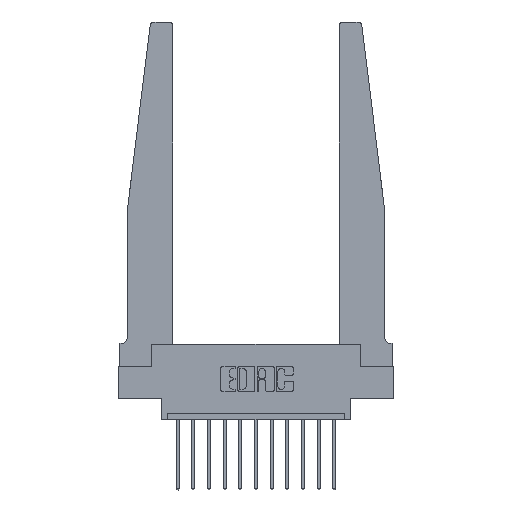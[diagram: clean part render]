
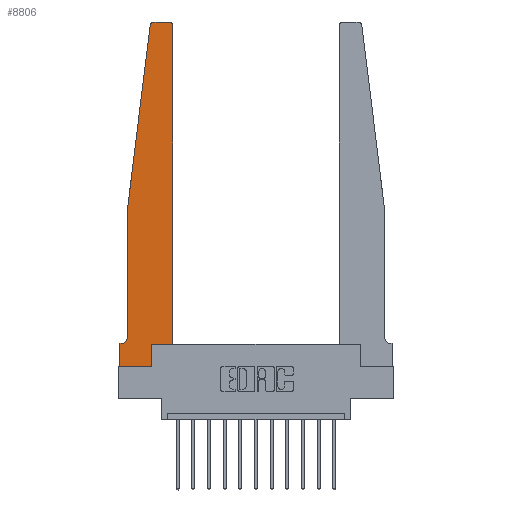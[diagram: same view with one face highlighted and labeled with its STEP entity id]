
A CAD part, top view. The second image highlights one B-rep face of the part: STEP entity #8806.
In plain terms, the highlighted planar face has unit normal (0, 0, 1).
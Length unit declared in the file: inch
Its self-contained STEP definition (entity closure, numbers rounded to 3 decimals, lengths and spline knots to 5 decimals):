
#67 = DIRECTION ( 'NONE',  ( 0., 0., -1. ) ) ;
#358 = CARTESIAN_POINT ( 'NONE',  ( 0.065, 1.25, 0.37 ) ) ;
#398 = CIRCLE ( 'NONE', #5786, 0.05 ) ;
#509 = PLANE ( 'NONE',  #15789 ) ;
#596 = CARTESIAN_POINT ( 'NONE',  ( 0.2605, 0., 0.37 ) ) ;
#938 = CARTESIAN_POINT ( 'NONE',  ( 0.24675, 2.72367, 0.37 ) ) ;
#985 = DIRECTION ( 'NONE',  ( 0., -1., 0. ) ) ;
#1071 = VERTEX_POINT ( 'NONE', #14875 ) ;
#1486 = EDGE_CURVE ( 'NONE', #5446, #10211, #9994, .T. ) ;
#1492 = LINE ( 'NONE', #4240, #8425 ) ;
#1549 = LINE ( 'NONE', #15722, #3857 ) ;
#1559 = ORIENTED_EDGE ( 'NONE', *, *, #1968, .T. ) ;
#1968 = EDGE_CURVE ( 'NONE', #2943, #9603, #1492, .T. ) ;
#2263 = VECTOR ( 'NONE', #5400, 39.37008 ) ;
#2424 = DIRECTION ( 'NONE',  ( 1., 0., 0. ) ) ;
#2767 = EDGE_CURVE ( 'NONE', #3061, #11729, #13934, .T. ) ;
#2943 = VERTEX_POINT ( 'NONE', #7527 ) ;
#2975 = DIRECTION ( 'NONE',  ( 1., 0., 0. ) ) ;
#3061 = VERTEX_POINT ( 'NONE', #358 ) ;
#3260 = ORIENTED_EDGE ( 'NONE', *, *, #6381, .T. ) ;
#3617 = EDGE_CURVE ( 'NONE', #9603, #7699, #12775, .T. ) ;
#3772 = DIRECTION ( 'NONE',  ( 0., 1., 0. ) ) ;
#3796 = CARTESIAN_POINT ( 'NONE',  ( 0.065, 1.25, 0.37 ) ) ;
#3857 = VECTOR ( 'NONE', #3772, 39.37008 ) ;
#3901 = VECTOR ( 'NONE', #14464, 39.37008 ) ;
#4104 = EDGE_CURVE ( 'NONE', #11659, #14454, #10845, .T. ) ;
#4240 = CARTESIAN_POINT ( 'NONE',  ( 0.25, 2.75, 0.37 ) ) ;
#4245 = DIRECTION ( 'NONE',  ( 0., 0., 1. ) ) ;
#4278 = EDGE_CURVE ( 'NONE', #10211, #7585, #8353, .T. ) ;
#4559 = CARTESIAN_POINT ( 'NONE',  ( 0., 0., 0.37 ) ) ;
#4719 = CARTESIAN_POINT ( 'NONE',  ( 0.395, 2.72, 0.37 ) ) ;
#4805 = ORIENTED_EDGE ( 'NONE', *, *, #1486, .T. ) ;
#4852 = CARTESIAN_POINT ( 'NONE',  ( 0.27653, 2.72, 0.37 ) ) ;
#5400 = DIRECTION ( 'NONE',  ( 0., 1., 0. ) ) ;
#5446 = VERTEX_POINT ( 'NONE', #596 ) ;
#5660 = EDGE_CURVE ( 'NONE', #7585, #1071, #1549, .T. ) ;
#5666 = VECTOR ( 'NONE', #985, 39.37008 ) ;
#5786 = AXIS2_PLACEMENT_3D ( 'NONE', #7438, #67, #6287 ) ;
#5827 = CARTESIAN_POINT ( 'NONE',  ( 0., 0., 0.37 ) ) ;
#5848 = VECTOR ( 'NONE', #15693, 39.37008 ) ;
#5949 = EDGE_LOOP ( 'NONE', ( #1559, #8254, #7114, #6825, #3260, #12101, #12035, #9757, #4805, #11507, #9281, #14024 ) ) ;
#5986 = DIRECTION ( 'NONE',  ( 1., 0., 0. ) ) ;
#6163 = DIRECTION ( 'NONE',  ( 0., 0., 1. ) ) ;
#6287 = DIRECTION ( 'NONE',  ( -1., 0., 0. ) ) ;
#6381 = EDGE_CURVE ( 'NONE', #11729, #9808, #398, .T. ) ;
#6825 = ORIENTED_EDGE ( 'NONE', *, *, #2767, .T. ) ;
#7023 = CARTESIAN_POINT ( 'NONE',  ( 0., 0., 0.37 ) ) ;
#7053 = EDGE_CURVE ( 'NONE', #1071, #2943, #12968, .T. ) ;
#7114 = ORIENTED_EDGE ( 'NONE', *, *, #9114, .T. ) ;
#7438 = CARTESIAN_POINT ( 'NONE',  ( 0.015, 0.2375, 0.37 ) ) ;
#7445 = VECTOR ( 'NONE', #7655, 39.37008 ) ;
#7527 = CARTESIAN_POINT ( 'NONE',  ( 0.395, 2.75, 0.37 ) ) ;
#7585 = VERTEX_POINT ( 'NONE', #11206 ) ;
#7655 = DIRECTION ( 'NONE',  ( -1., 0., 0. ) ) ;
#7699 = VERTEX_POINT ( 'NONE', #938 ) ;
#7885 = VECTOR ( 'NONE', #13179, 39.37008 ) ;
#8254 = ORIENTED_EDGE ( 'NONE', *, *, #3617, .T. ) ;
#8353 = LINE ( 'NONE', #14533, #3901 ) ;
#8425 = VECTOR ( 'NONE', #14144, 39.37008 ) ;
#8476 = CARTESIAN_POINT ( 'NONE',  ( 0.065, 0.2375, 0.37 ) ) ;
#8604 = DIRECTION ( 'NONE',  ( -0.122, -0.992, 0. ) ) ;
#8806 = ADVANCED_FACE ( 'NONE', ( #12799 ), #509, .T. ) ;
#9114 = EDGE_CURVE ( 'NONE', #7699, #3061, #13314, .T. ) ;
#9281 = ORIENTED_EDGE ( 'NONE', *, *, #5660, .T. ) ;
#9603 = VERTEX_POINT ( 'NONE', #13516 ) ;
#9718 = EDGE_CURVE ( 'NONE', #9808, #11659, #15323, .T. ) ;
#9757 = ORIENTED_EDGE ( 'NONE', *, *, #14555, .T. ) ;
#9808 = VERTEX_POINT ( 'NONE', #15416 ) ;
#9994 = LINE ( 'NONE', #12740, #2263 ) ;
#10052 = CARTESIAN_POINT ( 'NONE',  ( 0.065, 0.1875, 0.37 ) ) ;
#10211 = VERTEX_POINT ( 'NONE', #12782 ) ;
#10718 = AXIS2_PLACEMENT_3D ( 'NONE', #4719, #13348, #5986 ) ;
#10739 = CARTESIAN_POINT ( 'NONE',  ( 0.065, 1.25, 0.37 ) ) ;
#10829 = CARTESIAN_POINT ( 'NONE',  ( 0., 0.1875, 0.37 ) ) ;
#10845 = LINE ( 'NONE', #7023, #5666 ) ;
#11206 = CARTESIAN_POINT ( 'NONE',  ( 0.425, 0.18, 0.37 ) ) ;
#11507 = ORIENTED_EDGE ( 'NONE', *, *, #4278, .T. ) ;
#11609 = CARTESIAN_POINT ( 'NONE',  ( 0., 0.1875, 0.37 ) ) ;
#11659 = VERTEX_POINT ( 'NONE', #10829 ) ;
#11729 = VERTEX_POINT ( 'NONE', #8476 ) ;
#12035 = ORIENTED_EDGE ( 'NONE', *, *, #4104, .T. ) ;
#12101 = ORIENTED_EDGE ( 'NONE', *, *, #9718, .T. ) ;
#12438 = AXIS2_PLACEMENT_3D ( 'NONE', #4852, #6163, #2424 ) ;
#12740 = CARTESIAN_POINT ( 'NONE',  ( 0.2605, 0.18, 0.37 ) ) ;
#12775 = CIRCLE ( 'NONE', #12438, 0.03 ) ;
#12782 = CARTESIAN_POINT ( 'NONE',  ( 0.2605, 0.18, 0.37 ) ) ;
#12799 = FACE_OUTER_BOUND ( 'NONE', #5949, .T. ) ;
#12968 = CIRCLE ( 'NONE', #10718, 0.03 ) ;
#13179 = DIRECTION ( 'NONE',  ( 1., 0., 0. ) ) ;
#13314 = LINE ( 'NONE', #3796, #14448 ) ;
#13348 = DIRECTION ( 'NONE',  ( 0., 0., 1. ) ) ;
#13516 = CARTESIAN_POINT ( 'NONE',  ( 0.27653, 2.75, 0.37 ) ) ;
#13934 = LINE ( 'NONE', #10739, #5848 ) ;
#14024 = ORIENTED_EDGE ( 'NONE', *, *, #7053, .T. ) ;
#14144 = DIRECTION ( 'NONE',  ( -1., 0., 0. ) ) ;
#14448 = VECTOR ( 'NONE', #8604, 39.37008 ) ;
#14454 = VERTEX_POINT ( 'NONE', #5827 ) ;
#14464 = DIRECTION ( 'NONE',  ( 1., 0., 0. ) ) ;
#14533 = CARTESIAN_POINT ( 'NONE',  ( 0.425, 0.18, 0.37 ) ) ;
#14555 = EDGE_CURVE ( 'NONE', #14454, #5446, #14779, .T. ) ;
#14779 = LINE ( 'NONE', #4559, #7885 ) ;
#14875 = CARTESIAN_POINT ( 'NONE',  ( 0.425, 2.72, 0.37 ) ) ;
#15323 = LINE ( 'NONE', #10052, #7445 ) ;
#15416 = CARTESIAN_POINT ( 'NONE',  ( 0.015, 0.1875, 0.37 ) ) ;
#15693 = DIRECTION ( 'NONE',  ( 0., -1., 0. ) ) ;
#15722 = CARTESIAN_POINT ( 'NONE',  ( 0.425, 0.18, 0.37 ) ) ;
#15789 = AXIS2_PLACEMENT_3D ( 'NONE', #11609, #4245, #2975 ) ;
